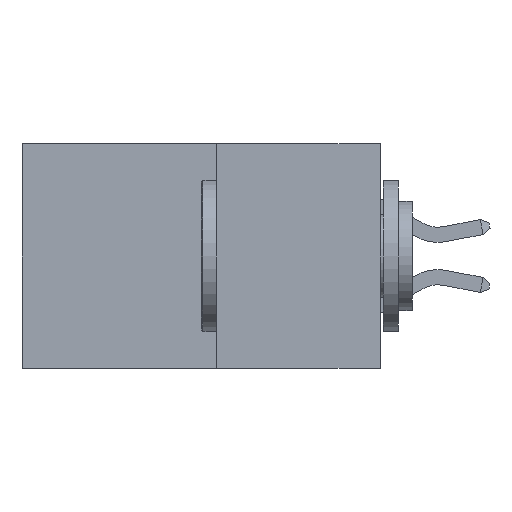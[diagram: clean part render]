
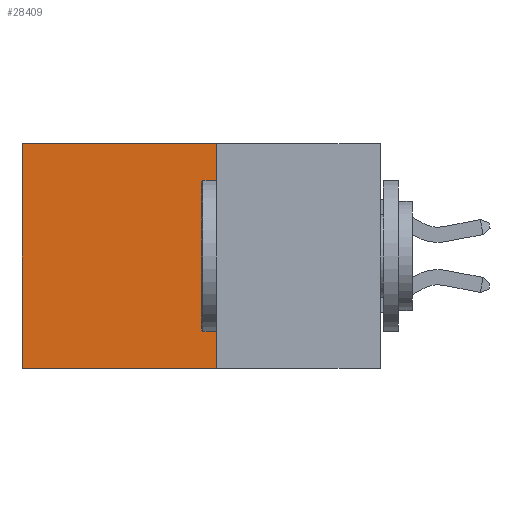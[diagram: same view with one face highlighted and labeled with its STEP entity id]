
A CAD part, left-side view. The second image highlights one B-rep face of the part: STEP entity #28409.
In plain terms, the highlighted planar face has unit normal (-1, 0, 0).
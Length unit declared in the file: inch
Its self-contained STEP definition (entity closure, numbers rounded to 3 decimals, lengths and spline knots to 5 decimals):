
#2632 = DIRECTION ( 'NONE',  ( 0., 0., -1. ) ) ;
#2813 = CARTESIAN_POINT ( 'NONE',  ( 0.277, 0.27, 0. ) ) ;
#4038 = VECTOR ( 'NONE', #7103, 39.37008 ) ;
#4502 = CARTESIAN_POINT ( 'NONE',  ( 0.277, 0.59, 0. ) ) ;
#5320 = DIRECTION ( 'NONE',  ( 0., 1., 0. ) ) ;
#5570 = LINE ( 'NONE', #26647, #28901 ) ;
#6213 = ORIENTED_EDGE ( 'NONE', *, *, #13517, .F. ) ;
#7073 = PLANE ( 'NONE',  #28764 ) ;
#7103 = DIRECTION ( 'NONE',  ( 0., 0., -1. ) ) ;
#7183 = EDGE_LOOP ( 'NONE', ( #9424, #28160, #6213, #19130 ) ) ;
#9051 = EDGE_CURVE ( 'NONE', #24446, #22956, #23985, .T. ) ;
#9319 = CARTESIAN_POINT ( 'NONE',  ( 0.277, 0.27, -0.37 ) ) ;
#9329 = VERTEX_POINT ( 'NONE', #22228 ) ;
#9424 = ORIENTED_EDGE ( 'NONE', *, *, #24954, .T. ) ;
#11682 = VERTEX_POINT ( 'NONE', #4502 ) ;
#12227 = CARTESIAN_POINT ( 'NONE',  ( 0.277, 0.27, -0.37 ) ) ;
#13053 = FACE_OUTER_BOUND ( 'NONE', #7183, .T. ) ;
#13517 = EDGE_CURVE ( 'NONE', #9329, #24446, #5570, .T. ) ;
#14350 = DIRECTION ( 'NONE',  ( 0., 1., 0. ) ) ;
#15431 = DIRECTION ( 'NONE',  ( 0., 0., -1. ) ) ;
#16355 = DIRECTION ( 'NONE',  ( 1., 0., 0. ) ) ;
#19130 = ORIENTED_EDGE ( 'NONE', *, *, #28478, .T. ) ;
#20352 = CARTESIAN_POINT ( 'NONE',  ( 0.277, 0.59, -0.37 ) ) ;
#20860 = CARTESIAN_POINT ( 'NONE',  ( 0.277, 0.27, -0.37 ) ) ;
#21619 = LINE ( 'NONE', #27541, #4038 ) ;
#22228 = CARTESIAN_POINT ( 'NONE',  ( 0.277, 0.27, 0. ) ) ;
#22371 = VECTOR ( 'NONE', #14350, 39.37008 ) ;
#22956 = VERTEX_POINT ( 'NONE', #20352 ) ;
#23985 = LINE ( 'NONE', #12227, #29098 ) ;
#24446 = VERTEX_POINT ( 'NONE', #9319 ) ;
#24954 = EDGE_CURVE ( 'NONE', #11682, #22956, #21619, .T. ) ;
#26647 = CARTESIAN_POINT ( 'NONE',  ( 0.277, 0.27, -0.37 ) ) ;
#27541 = CARTESIAN_POINT ( 'NONE',  ( 0.277, 0.59, -0.37 ) ) ;
#28160 = ORIENTED_EDGE ( 'NONE', *, *, #9051, .F. ) ;
#28409 = ADVANCED_FACE ( 'NONE', ( #13053 ), #7073, .F. ) ;
#28478 = EDGE_CURVE ( 'NONE', #9329, #11682, #28867, .T. ) ;
#28764 = AXIS2_PLACEMENT_3D ( 'NONE', #20860, #16355, #2632 ) ;
#28867 = LINE ( 'NONE', #2813, #22371 ) ;
#28901 = VECTOR ( 'NONE', #15431, 39.37008 ) ;
#29098 = VECTOR ( 'NONE', #5320, 39.37008 ) ;
